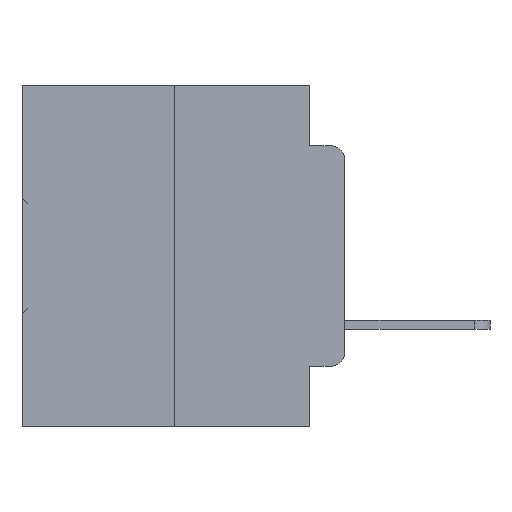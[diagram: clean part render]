
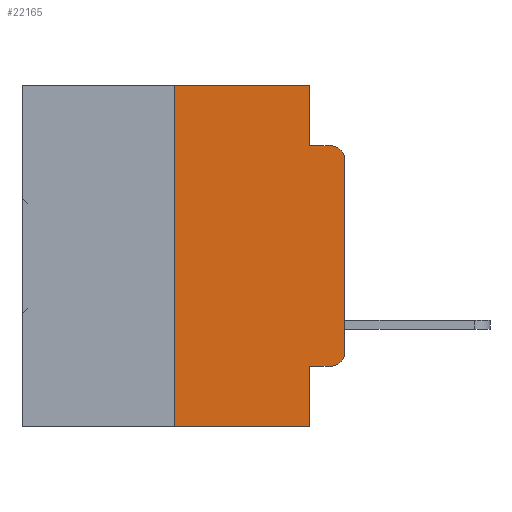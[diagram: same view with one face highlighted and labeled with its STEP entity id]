
A CAD part, left-side view. The second image highlights one B-rep face of the part: STEP entity #22165.
In plain terms, the highlighted planar face has unit normal (-1, 0, 0).
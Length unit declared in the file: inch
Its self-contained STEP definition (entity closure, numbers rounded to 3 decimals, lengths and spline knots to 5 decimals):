
#91 = EDGE_CURVE ( 'NONE', #1996, #2412, #16393, .T. ) ;
#146 = ORIENTED_EDGE ( 'NONE', *, *, #3437, .F. ) ;
#1563 = VECTOR ( 'NONE', #14051, 39.37008 ) ;
#1870 = EDGE_CURVE ( 'NONE', #27835, #17019, #24615, .T. ) ;
#1996 = VERTEX_POINT ( 'NONE', #19781 ) ;
#2093 = VERTEX_POINT ( 'NONE', #4981 ) ;
#2412 = VERTEX_POINT ( 'NONE', #4568 ) ;
#2417 = DIRECTION ( 'NONE',  ( 0., 0., -1. ) ) ;
#2658 = VECTOR ( 'NONE', #33146, 39.37008 ) ;
#3437 = EDGE_CURVE ( 'NONE', #14267, #2093, #16881, .T. ) ;
#3685 = CARTESIAN_POINT ( 'NONE',  ( 0., 0.051, -0.4115 ) ) ;
#4185 = VECTOR ( 'NONE', #16148, 39.37008 ) ;
#4568 = CARTESIAN_POINT ( 'NONE',  ( 0., 0.051, -0.5 ) ) ;
#4943 = ORIENTED_EDGE ( 'NONE', *, *, #18472, .F. ) ;
#4981 = CARTESIAN_POINT ( 'NONE',  ( 0., 0.051, 0. ) ) ;
#7271 = LINE ( 'NONE', #12082, #34999 ) ;
#7822 = DIRECTION ( 'NONE',  ( 0., 0., -1. ) ) ;
#8299 = AXIS2_PLACEMENT_3D ( 'NONE', #10531, #29404, #13350 ) ;
#8313 = FACE_OUTER_BOUND ( 'NONE', #28051, .T. ) ;
#9927 = AXIS2_PLACEMENT_3D ( 'NONE', #19482, #14062, #32737 ) ;
#10383 = VECTOR ( 'NONE', #22169, 39.37008 ) ;
#10448 = CARTESIAN_POINT ( 'NONE',  ( 0., 0.051, 0. ) ) ;
#10531 = CARTESIAN_POINT ( 'NONE',  ( 0., 0.02, -0.1085 ) ) ;
#10540 = VERTEX_POINT ( 'NONE', #13059 ) ;
#11241 = EDGE_CURVE ( 'NONE', #27835, #2412, #31778, .T. ) ;
#11973 = CARTESIAN_POINT ( 'NONE',  ( 0., 0.473, -0.5 ) ) ;
#12082 = CARTESIAN_POINT ( 'NONE',  ( 0., 0., 0. ) ) ;
#12480 = CARTESIAN_POINT ( 'NONE',  ( 0., 0.051, -0.0885 ) ) ;
#12502 = CARTESIAN_POINT ( 'NONE',  ( 0., 0., -0.1085 ) ) ;
#12650 = CIRCLE ( 'NONE', #24788, 0.02 ) ;
#12744 = VECTOR ( 'NONE', #16187, 39.37008 ) ;
#13059 = CARTESIAN_POINT ( 'NONE',  ( 0., 0., -0.3915 ) ) ;
#13350 = DIRECTION ( 'NONE',  ( 0., 0., -1. ) ) ;
#14051 = DIRECTION ( 'NONE',  ( 0., -1., 0. ) ) ;
#14062 = DIRECTION ( 'NONE',  ( 1., 0., 0. ) ) ;
#14267 = VERTEX_POINT ( 'NONE', #18261 ) ;
#14549 = LINE ( 'NONE', #34284, #20120 ) ;
#14716 = DIRECTION ( 'NONE',  ( 0., 0., 1. ) ) ;
#15378 = ORIENTED_EDGE ( 'NONE', *, *, #11241, .F. ) ;
#15488 = CARTESIAN_POINT ( 'NONE',  ( 0., 0.02, -0.0885 ) ) ;
#15538 = CIRCLE ( 'NONE', #8299, 0.02 ) ;
#15695 = DIRECTION ( 'NONE',  ( 0., 0., 1. ) ) ;
#16148 = DIRECTION ( 'NONE',  ( 0., -1., 0. ) ) ;
#16187 = DIRECTION ( 'NONE',  ( 0., 0., -1. ) ) ;
#16393 = LINE ( 'NONE', #11973, #1563 ) ;
#16881 = LINE ( 'NONE', #21929, #10383 ) ;
#17019 = VERTEX_POINT ( 'NONE', #28308 ) ;
#17494 = ORIENTED_EDGE ( 'NONE', *, *, #32399, .T. ) ;
#17808 = VERTEX_POINT ( 'NONE', #15488 ) ;
#18261 = CARTESIAN_POINT ( 'NONE',  ( 0., 0.25, 0. ) ) ;
#18472 = EDGE_CURVE ( 'NONE', #2093, #30837, #27121, .T. ) ;
#18783 = CARTESIAN_POINT ( 'NONE',  ( 0., 0.051, -0.0885 ) ) ;
#18950 = CARTESIAN_POINT ( 'NONE',  ( 0., 0.051, 0. ) ) ;
#19018 = DIRECTION ( 'NONE',  ( -1., 0., 0. ) ) ;
#19482 = CARTESIAN_POINT ( 'NONE',  ( 0., 0.473, 0. ) ) ;
#19676 = ORIENTED_EDGE ( 'NONE', *, *, #1870, .T. ) ;
#19781 = CARTESIAN_POINT ( 'NONE',  ( 0., 0.25, -0.5 ) ) ;
#20120 = VECTOR ( 'NONE', #15695, 39.37008 ) ;
#21358 = ORIENTED_EDGE ( 'NONE', *, *, #22050, .T. ) ;
#21929 = CARTESIAN_POINT ( 'NONE',  ( 0., 0.473, 0. ) ) ;
#22050 = EDGE_CURVE ( 'NONE', #17019, #10540, #12650, .T. ) ;
#22165 = ADVANCED_FACE ( 'NONE', ( #8313 ), #24897, .F. ) ;
#22169 = DIRECTION ( 'NONE',  ( 0., -1., 0. ) ) ;
#24300 = ORIENTED_EDGE ( 'NONE', *, *, #25854, .F. ) ;
#24615 = LINE ( 'NONE', #3685, #2658 ) ;
#24788 = AXIS2_PLACEMENT_3D ( 'NONE', #34796, #19018, #2417 ) ;
#24877 = VECTOR ( 'NONE', #7822, 39.37008 ) ;
#24897 = PLANE ( 'NONE',  #9927 ) ;
#25519 = ORIENTED_EDGE ( 'NONE', *, *, #29288, .F. ) ;
#25854 = EDGE_CURVE ( 'NONE', #30837, #17808, #26036, .T. ) ;
#26036 = LINE ( 'NONE', #18783, #4185 ) ;
#26268 = VERTEX_POINT ( 'NONE', #12502 ) ;
#26302 = ORIENTED_EDGE ( 'NONE', *, *, #31532, .T. ) ;
#27121 = LINE ( 'NONE', #18950, #12744 ) ;
#27178 = ORIENTED_EDGE ( 'NONE', *, *, #91, .T. ) ;
#27835 = VERTEX_POINT ( 'NONE', #29468 ) ;
#28051 = EDGE_LOOP ( 'NONE', ( #17494, #26302, #24300, #4943, #146, #25519, #27178, #15378, #19676, #21358 ) ) ;
#28308 = CARTESIAN_POINT ( 'NONE',  ( 0., 0.02, -0.4115 ) ) ;
#29288 = EDGE_CURVE ( 'NONE', #1996, #14267, #14549, .T. ) ;
#29404 = DIRECTION ( 'NONE',  ( -1., 0., 0. ) ) ;
#29468 = CARTESIAN_POINT ( 'NONE',  ( 0., 0.051, -0.4115 ) ) ;
#30837 = VERTEX_POINT ( 'NONE', #12480 ) ;
#31532 = EDGE_CURVE ( 'NONE', #26268, #17808, #15538, .T. ) ;
#31778 = LINE ( 'NONE', #10448, #24877 ) ;
#32399 = EDGE_CURVE ( 'NONE', #10540, #26268, #7271, .T. ) ;
#32737 = DIRECTION ( 'NONE',  ( 0., 0., -1. ) ) ;
#33146 = DIRECTION ( 'NONE',  ( 0., -1., 0. ) ) ;
#34284 = CARTESIAN_POINT ( 'NONE',  ( 0., 0.25, 0. ) ) ;
#34796 = CARTESIAN_POINT ( 'NONE',  ( 0., 0.02, -0.3915 ) ) ;
#34999 = VECTOR ( 'NONE', #14716, 39.37008 ) ;
